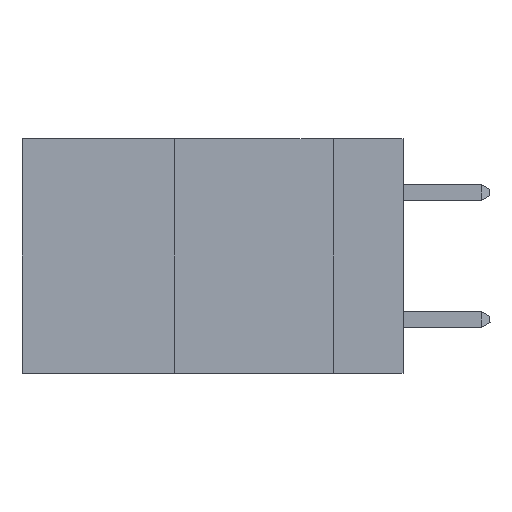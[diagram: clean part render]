
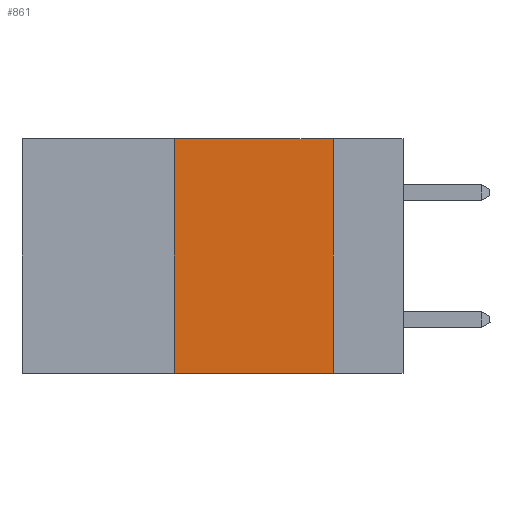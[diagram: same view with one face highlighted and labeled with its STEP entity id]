
A CAD part, left-side view. The second image highlights one B-rep face of the part: STEP entity #861.
In plain terms, the highlighted planar face has unit normal (-1, 0, 0).
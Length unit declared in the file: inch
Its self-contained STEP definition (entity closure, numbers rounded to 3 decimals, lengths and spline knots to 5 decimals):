
#861 = ADVANCED_FACE ( 'NONE', ( #12701 ), #5802, .F. ) ;
#1176 = VECTOR ( 'NONE', #8173, 39.37008 ) ;
#2264 = CARTESIAN_POINT ( 'NONE',  ( 0., 0.11, -0.37 ) ) ;
#3000 = VERTEX_POINT ( 'NONE', #2264 ) ;
#4007 = AXIS2_PLACEMENT_3D ( 'NONE', #4181, #12993, #19871 ) ;
#4181 = CARTESIAN_POINT ( 'NONE',  ( 0., 0.6, 0. ) ) ;
#4498 = CARTESIAN_POINT ( 'NONE',  ( 0., 0.36, 0. ) ) ;
#4525 = VECTOR ( 'NONE', #7906, 39.37008 ) ;
#5237 = VERTEX_POINT ( 'NONE', #13753 ) ;
#5602 = VECTOR ( 'NONE', #10677, 39.37008 ) ;
#5802 = PLANE ( 'NONE',  #4007 ) ;
#5811 = LINE ( 'NONE', #4498, #1176 ) ;
#6087 = LINE ( 'NONE', #22003, #21917 ) ;
#6130 = DIRECTION ( 'NONE',  ( 0., -1., 0. ) ) ;
#6185 = LINE ( 'NONE', #8937, #5602 ) ;
#7043 = ORIENTED_EDGE ( 'NONE', *, *, #14108, .F. ) ;
#7906 = DIRECTION ( 'NONE',  ( 0., 0., -1. ) ) ;
#8173 = DIRECTION ( 'NONE',  ( 0., 0., 1. ) ) ;
#8469 = VERTEX_POINT ( 'NONE', #16629 ) ;
#8890 = VERTEX_POINT ( 'NONE', #16442 ) ;
#8937 = CARTESIAN_POINT ( 'NONE',  ( 0., 0.6, -0.37 ) ) ;
#9147 = LINE ( 'NONE', #13409, #4525 ) ;
#9528 = EDGE_LOOP ( 'NONE', ( #16975, #14580, #7043, #14427 ) ) ;
#10677 = DIRECTION ( 'NONE',  ( 0., -1., 0. ) ) ;
#12701 = FACE_OUTER_BOUND ( 'NONE', #9528, .T. ) ;
#12993 = DIRECTION ( 'NONE',  ( 1., 0., 0. ) ) ;
#13409 = CARTESIAN_POINT ( 'NONE',  ( 0., 0.11, 0. ) ) ;
#13753 = CARTESIAN_POINT ( 'NONE',  ( 0., 0.36, 0. ) ) ;
#14108 = EDGE_CURVE ( 'NONE', #8890, #5237, #5811, .T. ) ;
#14427 = ORIENTED_EDGE ( 'NONE', *, *, #15802, .T. ) ;
#14580 = ORIENTED_EDGE ( 'NONE', *, *, #20058, .F. ) ;
#15802 = EDGE_CURVE ( 'NONE', #8890, #3000, #6185, .T. ) ;
#16442 = CARTESIAN_POINT ( 'NONE',  ( 0., 0.36, -0.37 ) ) ;
#16629 = CARTESIAN_POINT ( 'NONE',  ( 0., 0.11, 0. ) ) ;
#16975 = ORIENTED_EDGE ( 'NONE', *, *, #18440, .F. ) ;
#18440 = EDGE_CURVE ( 'NONE', #8469, #3000, #9147, .T. ) ;
#19871 = DIRECTION ( 'NONE',  ( 0., 0., -1. ) ) ;
#20058 = EDGE_CURVE ( 'NONE', #5237, #8469, #6087, .T. ) ;
#21917 = VECTOR ( 'NONE', #6130, 39.37008 ) ;
#22003 = CARTESIAN_POINT ( 'NONE',  ( 0., 0.6, 0. ) ) ;
